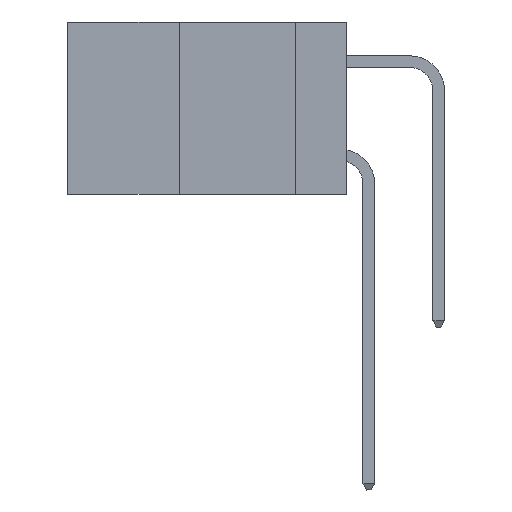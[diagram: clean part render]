
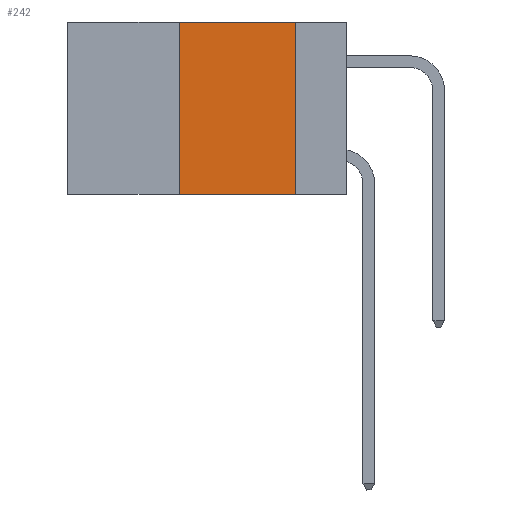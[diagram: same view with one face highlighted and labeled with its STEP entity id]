
A CAD part, left-side view. The second image highlights one B-rep face of the part: STEP entity #242.
In plain terms, the highlighted planar face has unit normal (-1, 0, 0).
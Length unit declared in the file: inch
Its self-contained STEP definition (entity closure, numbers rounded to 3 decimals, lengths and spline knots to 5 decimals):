
#242 = ADVANCED_FACE ( 'NONE', ( #637 ), #10386, .F. ) ;
#637 = FACE_OUTER_BOUND ( 'NONE', #797, .T. ) ;
#797 = EDGE_LOOP ( 'NONE', ( #12457, #12007, #6598, #9893 ) ) ;
#1233 = EDGE_CURVE ( 'NONE', #2900, #10788, #12986, .T. ) ;
#1248 = VECTOR ( 'NONE', #1829, 39.37008 ) ;
#1284 = EDGE_CURVE ( 'NONE', #2900, #1724, #7820, .T. ) ;
#1295 = DIRECTION ( 'NONE',  ( 0., 0., -1. ) ) ;
#1724 = VERTEX_POINT ( 'NONE', #3665 ) ;
#1759 = EDGE_CURVE ( 'NONE', #10788, #7025, #2543, .T. ) ;
#1829 = DIRECTION ( 'NONE',  ( 0., 0., 1. ) ) ;
#2543 = LINE ( 'NONE', #7861, #3991 ) ;
#2900 = VERTEX_POINT ( 'NONE', #13121 ) ;
#3665 = CARTESIAN_POINT ( 'NONE',  ( 0., 0.11, -0.37 ) ) ;
#3991 = VECTOR ( 'NONE', #10805, 39.37008 ) ;
#4862 = VECTOR ( 'NONE', #1295, 39.37008 ) ;
#6598 = ORIENTED_EDGE ( 'NONE', *, *, #1233, .F. ) ;
#7025 = VERTEX_POINT ( 'NONE', #12412 ) ;
#7069 = CARTESIAN_POINT ( 'NONE',  ( 0., 0.6, -0.37 ) ) ;
#7587 = LINE ( 'NONE', #12772, #4862 ) ;
#7820 = LINE ( 'NONE', #7069, #9129 ) ;
#7861 = CARTESIAN_POINT ( 'NONE',  ( 0., 0.6, 0. ) ) ;
#8312 = CARTESIAN_POINT ( 'NONE',  ( 0., 0.6, 0. ) ) ;
#9129 = VECTOR ( 'NONE', #10450, 39.37008 ) ;
#9155 = CARTESIAN_POINT ( 'NONE',  ( 0., 0.36, 0. ) ) ;
#9311 = DIRECTION ( 'NONE',  ( 0., 0., -1. ) ) ;
#9893 = ORIENTED_EDGE ( 'NONE', *, *, #1284, .T. ) ;
#10386 = PLANE ( 'NONE',  #12879 ) ;
#10450 = DIRECTION ( 'NONE',  ( 0., -1., 0. ) ) ;
#10788 = VERTEX_POINT ( 'NONE', #11558 ) ;
#10805 = DIRECTION ( 'NONE',  ( 0., -1., 0. ) ) ;
#11423 = DIRECTION ( 'NONE',  ( 1., 0., 0. ) ) ;
#11442 = EDGE_CURVE ( 'NONE', #7025, #1724, #7587, .T. ) ;
#11558 = CARTESIAN_POINT ( 'NONE',  ( 0., 0.36, 0. ) ) ;
#12007 = ORIENTED_EDGE ( 'NONE', *, *, #1759, .F. ) ;
#12412 = CARTESIAN_POINT ( 'NONE',  ( 0., 0.11, 0. ) ) ;
#12457 = ORIENTED_EDGE ( 'NONE', *, *, #11442, .F. ) ;
#12772 = CARTESIAN_POINT ( 'NONE',  ( 0., 0.11, 0. ) ) ;
#12879 = AXIS2_PLACEMENT_3D ( 'NONE', #8312, #11423, #9311 ) ;
#12986 = LINE ( 'NONE', #9155, #1248 ) ;
#13121 = CARTESIAN_POINT ( 'NONE',  ( 0., 0.36, -0.37 ) ) ;
